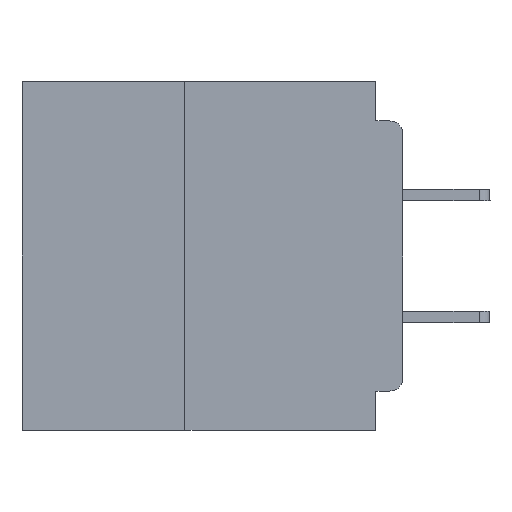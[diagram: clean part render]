
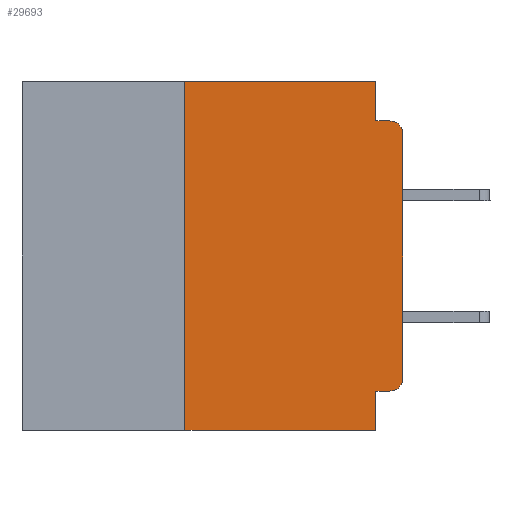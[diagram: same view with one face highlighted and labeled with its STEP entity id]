
A CAD part, left-side view. The second image highlights one B-rep face of the part: STEP entity #29693.
In plain terms, the highlighted planar face has unit normal (-1, 0, 0).
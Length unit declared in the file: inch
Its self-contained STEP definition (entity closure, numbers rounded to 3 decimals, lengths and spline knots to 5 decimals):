
#112 = LINE ( 'NONE', #27806, #26163 ) ;
#873 = CARTESIAN_POINT ( 'NONE',  ( 0., 0.031, -0.4 ) ) ;
#1536 = AXIS2_PLACEMENT_3D ( 'NONE', #27286, #63410, #32464 ) ;
#1786 = VERTEX_POINT ( 'NONE', #62993 ) ;
#1845 = AXIS2_PLACEMENT_3D ( 'NONE', #12997, #49170, #18214 ) ;
#3759 = ORIENTED_EDGE ( 'NONE', *, *, #17427, .F. ) ;
#3861 = EDGE_CURVE ( 'NONE', #35396, #65092, #112, .T. ) ;
#5106 = CARTESIAN_POINT ( 'NONE',  ( 0., 0., -0.355 ) ) ;
#5530 = EDGE_CURVE ( 'NONE', #1786, #9385, #34967, .T. ) ;
#6813 = EDGE_CURVE ( 'NONE', #65245, #42236, #10474, .T. ) ;
#6876 = DIRECTION ( 'NONE',  ( 1., 0., 0. ) ) ;
#7157 = DIRECTION ( 'NONE',  ( 0., 0., 1. ) ) ;
#9385 = VERTEX_POINT ( 'NONE', #35590 ) ;
#10037 = LINE ( 'NONE', #29189, #63390 ) ;
#10474 = LINE ( 'NONE', #12828, #24266 ) ;
#12093 = VERTEX_POINT ( 'NONE', #60541 ) ;
#12624 = ORIENTED_EDGE ( 'NONE', *, *, #65772, .T. ) ;
#12828 = CARTESIAN_POINT ( 'NONE',  ( 0., 0., -0.045 ) ) ;
#12997 = CARTESIAN_POINT ( 'NONE',  ( 0., 0.015, -0.34 ) ) ;
#13018 = ORIENTED_EDGE ( 'NONE', *, *, #50289, .F. ) ;
#14604 = ORIENTED_EDGE ( 'NONE', *, *, #5530, .T. ) ;
#15984 = ORIENTED_EDGE ( 'NONE', *, *, #3861, .F. ) ;
#16886 = DIRECTION ( 'NONE',  ( 0., -1., 0. ) ) ;
#17427 = EDGE_CURVE ( 'NONE', #40212, #65245, #10037, .T. ) ;
#17553 = VECTOR ( 'NONE', #30857, 39.37008 ) ;
#18214 = DIRECTION ( 'NONE',  ( 0., 0., -1. ) ) ;
#18276 = CARTESIAN_POINT ( 'NONE',  ( 0., 0.031, 0. ) ) ;
#21076 = LINE ( 'NONE', #23918, #48561 ) ;
#21100 = VECTOR ( 'NONE', #16886, 39.37008 ) ;
#22518 = FACE_OUTER_BOUND ( 'NONE', #57379, .T. ) ;
#23720 = EDGE_CURVE ( 'NONE', #65092, #40212, #50186, .T. ) ;
#23918 = CARTESIAN_POINT ( 'NONE',  ( 0., 0.437, -0.4 ) ) ;
#24266 = VECTOR ( 'NONE', #43855, 39.37008 ) ;
#24632 = ORIENTED_EDGE ( 'NONE', *, *, #23720, .F. ) ;
#26163 = VECTOR ( 'NONE', #7157, 39.37008 ) ;
#26268 = ORIENTED_EDGE ( 'NONE', *, *, #28986, .T. ) ;
#26639 = VERTEX_POINT ( 'NONE', #45704 ) ;
#27275 = CARTESIAN_POINT ( 'NONE',  ( 0., 0.437, 0. ) ) ;
#27286 = CARTESIAN_POINT ( 'NONE',  ( 0., 0.015, -0.06 ) ) ;
#27806 = CARTESIAN_POINT ( 'NONE',  ( 0., 0.25, -0.4 ) ) ;
#28986 = EDGE_CURVE ( 'NONE', #9385, #12093, #36251, .T. ) ;
#29189 = CARTESIAN_POINT ( 'NONE',  ( 0., 0.031, 0. ) ) ;
#29693 = ADVANCED_FACE ( 'NONE', ( #22518 ), #58494, .F. ) ;
#30857 = DIRECTION ( 'NONE',  ( 0., 0., -1. ) ) ;
#30968 = DIRECTION ( 'NONE',  ( 0., 1., 0. ) ) ;
#31008 = LINE ( 'NONE', #5106, #58507 ) ;
#32464 = DIRECTION ( 'NONE',  ( 0., 0., -1. ) ) ;
#32488 = CARTESIAN_POINT ( 'NONE',  ( 0., 0.437, 0. ) ) ;
#33219 = CARTESIAN_POINT ( 'NONE',  ( 0., 0.031, -0.045 ) ) ;
#34438 = VERTEX_POINT ( 'NONE', #873 ) ;
#34967 = CIRCLE ( 'NONE', #1845, 0.015 ) ;
#35396 = VERTEX_POINT ( 'NONE', #44602 ) ;
#35590 = CARTESIAN_POINT ( 'NONE',  ( 0., 0., -0.34 ) ) ;
#36251 = LINE ( 'NONE', #36660, #49977 ) ;
#36660 = CARTESIAN_POINT ( 'NONE',  ( 0., 0., 0. ) ) ;
#38106 = EDGE_CURVE ( 'NONE', #1786, #26639, #31008, .T. ) ;
#40212 = VERTEX_POINT ( 'NONE', #18276 ) ;
#41879 = DIRECTION ( 'NONE',  ( 0., 0., 1. ) ) ;
#42236 = VERTEX_POINT ( 'NONE', #65471 ) ;
#42325 = CARTESIAN_POINT ( 'NONE',  ( 0., 0.25, 0. ) ) ;
#43145 = DIRECTION ( 'NONE',  ( 0., 0., -1. ) ) ;
#43207 = ORIENTED_EDGE ( 'NONE', *, *, #38106, .F. ) ;
#43855 = DIRECTION ( 'NONE',  ( 0., -1., 0. ) ) ;
#44525 = ORIENTED_EDGE ( 'NONE', *, *, #6813, .F. ) ;
#44602 = CARTESIAN_POINT ( 'NONE',  ( 0., 0.25, -0.4 ) ) ;
#45704 = CARTESIAN_POINT ( 'NONE',  ( 0., 0.031, -0.355 ) ) ;
#48561 = VECTOR ( 'NONE', #54879, 39.37008 ) ;
#49170 = DIRECTION ( 'NONE',  ( -1., 0., 0. ) ) ;
#49977 = VECTOR ( 'NONE', #41879, 39.37008 ) ;
#50186 = LINE ( 'NONE', #27275, #21100 ) ;
#50289 = EDGE_CURVE ( 'NONE', #26639, #34438, #58798, .T. ) ;
#50910 = AXIS2_PLACEMENT_3D ( 'NONE', #32488, #6876, #43145 ) ;
#54879 = DIRECTION ( 'NONE',  ( 0., -1., 0. ) ) ;
#56415 = ORIENTED_EDGE ( 'NONE', *, *, #57228, .T. ) ;
#56609 = CARTESIAN_POINT ( 'NONE',  ( 0., 0.031, -0.4 ) ) ;
#57228 = EDGE_CURVE ( 'NONE', #35396, #34438, #21076, .T. ) ;
#57379 = EDGE_LOOP ( 'NONE', ( #26268, #12624, #44525, #3759, #24632, #15984, #56415, #13018, #43207, #14604 ) ) ;
#58494 = PLANE ( 'NONE',  #50910 ) ;
#58507 = VECTOR ( 'NONE', #30968, 39.37008 ) ;
#58798 = LINE ( 'NONE', #56609, #17553 ) ;
#60153 = DIRECTION ( 'NONE',  ( 0., 0., -1. ) ) ;
#60541 = CARTESIAN_POINT ( 'NONE',  ( 0., 0., -0.06 ) ) ;
#60874 = CIRCLE ( 'NONE', #1536, 0.015 ) ;
#62993 = CARTESIAN_POINT ( 'NONE',  ( 0., 0.015, -0.355 ) ) ;
#63390 = VECTOR ( 'NONE', #60153, 39.37008 ) ;
#63410 = DIRECTION ( 'NONE',  ( -1., 0., 0. ) ) ;
#65092 = VERTEX_POINT ( 'NONE', #42325 ) ;
#65245 = VERTEX_POINT ( 'NONE', #33219 ) ;
#65471 = CARTESIAN_POINT ( 'NONE',  ( 0., 0.015, -0.045 ) ) ;
#65772 = EDGE_CURVE ( 'NONE', #12093, #42236, #60874, .T. ) ;
